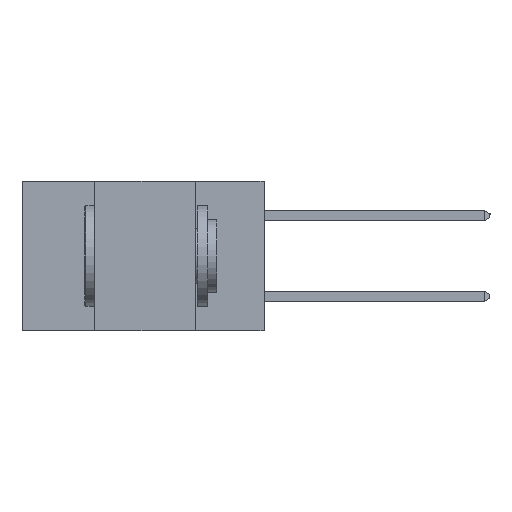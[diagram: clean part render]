
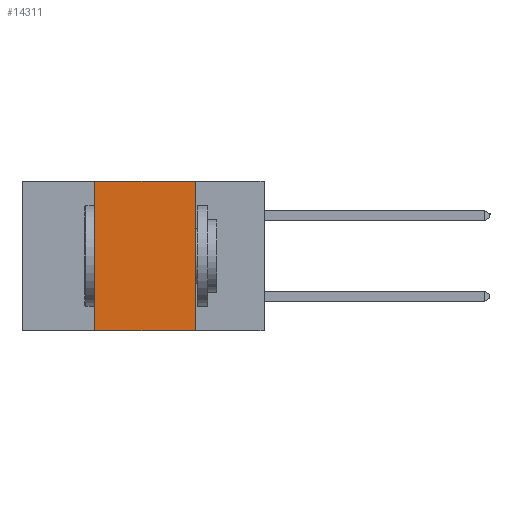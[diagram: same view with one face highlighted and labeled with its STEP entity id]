
A CAD part, left-side view. The second image highlights one B-rep face of the part: STEP entity #14311.
In plain terms, the highlighted planar face has unit normal (-1, 0, 0).
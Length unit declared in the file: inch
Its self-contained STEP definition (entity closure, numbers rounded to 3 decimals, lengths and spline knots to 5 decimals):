
#1 = EDGE_CURVE ( 'NONE', #2130, #11247, #713, .T. ) ;
#713 = LINE ( 'NONE', #7384, #12954 ) ;
#779 = DIRECTION ( 'NONE',  ( 0., -1., 0. ) ) ;
#875 = CARTESIAN_POINT ( 'NONE',  ( 0., 0.17, 0. ) ) ;
#1354 = VERTEX_POINT ( 'NONE', #1596 ) ;
#1520 = ORIENTED_EDGE ( 'NONE', *, *, #1794, .F. ) ;
#1596 = CARTESIAN_POINT ( 'NONE',  ( 0., 0.17, -0.37 ) ) ;
#1794 = EDGE_CURVE ( 'NONE', #13539, #1354, #14120, .T. ) ;
#2130 = VERTEX_POINT ( 'NONE', #8079 ) ;
#2356 = PLANE ( 'NONE',  #3457 ) ;
#2685 = CARTESIAN_POINT ( 'NONE',  ( 0., 0.17, -0.37 ) ) ;
#3457 = AXIS2_PLACEMENT_3D ( 'NONE', #12458, #10037, #8936 ) ;
#4165 = LINE ( 'NONE', #8753, #4324 ) ;
#4324 = VECTOR ( 'NONE', #779, 39.37008 ) ;
#4629 = CARTESIAN_POINT ( 'NONE',  ( 0., 0.42, 0. ) ) ;
#4721 = VECTOR ( 'NONE', #12941, 39.37008 ) ;
#5157 = VECTOR ( 'NONE', #7577, 39.37008 ) ;
#5162 = ORIENTED_EDGE ( 'NONE', *, *, #7517, .F. ) ;
#5181 = ORIENTED_EDGE ( 'NONE', *, *, #9372, .T. ) ;
#5569 = FACE_OUTER_BOUND ( 'NONE', #11156, .T. ) ;
#7227 = ORIENTED_EDGE ( 'NONE', *, *, #1, .F. ) ;
#7229 = DIRECTION ( 'NONE',  ( 0., 0., 1. ) ) ;
#7384 = CARTESIAN_POINT ( 'NONE',  ( 0., 0.42, -0.37 ) ) ;
#7517 = EDGE_CURVE ( 'NONE', #11247, #13539, #8367, .T. ) ;
#7577 = DIRECTION ( 'NONE',  ( 0., -1., 0. ) ) ;
#8079 = CARTESIAN_POINT ( 'NONE',  ( 0., 0.42, -0.37 ) ) ;
#8367 = LINE ( 'NONE', #12857, #5157 ) ;
#8753 = CARTESIAN_POINT ( 'NONE',  ( 0., 0.6, -0.37 ) ) ;
#8936 = DIRECTION ( 'NONE',  ( 0., 0., -1. ) ) ;
#9372 = EDGE_CURVE ( 'NONE', #2130, #1354, #4165, .T. ) ;
#10037 = DIRECTION ( 'NONE',  ( 1., 0., 0. ) ) ;
#11156 = EDGE_LOOP ( 'NONE', ( #1520, #5162, #7227, #5181 ) ) ;
#11247 = VERTEX_POINT ( 'NONE', #4629 ) ;
#12458 = CARTESIAN_POINT ( 'NONE',  ( 0., 0.6, 0. ) ) ;
#12857 = CARTESIAN_POINT ( 'NONE',  ( 0., 0.6, 0. ) ) ;
#12941 = DIRECTION ( 'NONE',  ( 0., 0., -1. ) ) ;
#12954 = VECTOR ( 'NONE', #7229, 39.37008 ) ;
#13539 = VERTEX_POINT ( 'NONE', #875 ) ;
#14120 = LINE ( 'NONE', #2685, #4721 ) ;
#14311 = ADVANCED_FACE ( 'NONE', ( #5569 ), #2356, .F. ) ;
